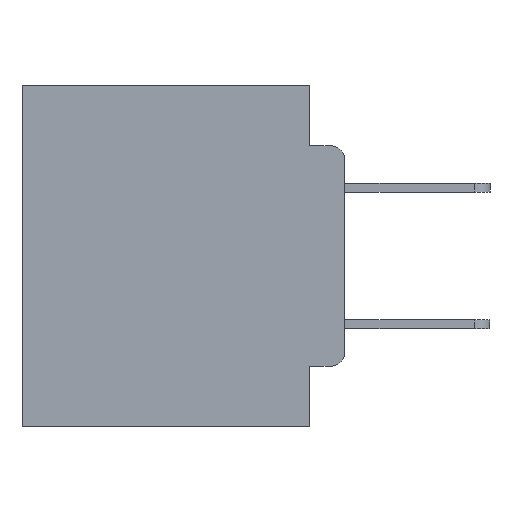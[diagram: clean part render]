
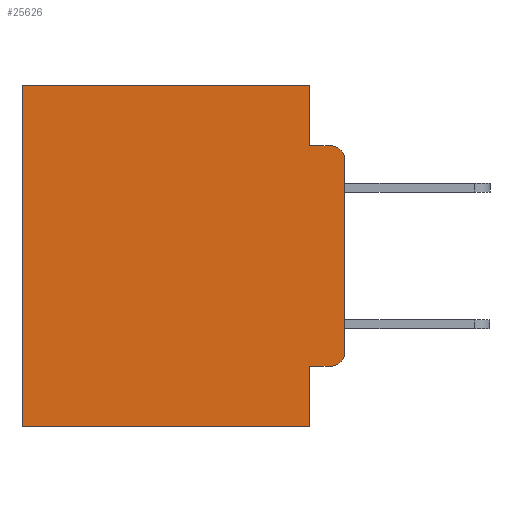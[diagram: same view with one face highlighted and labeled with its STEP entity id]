
A CAD part, left-side view. The second image highlights one B-rep face of the part: STEP entity #25626.
In plain terms, the highlighted planar face has unit normal (-1, 0, 0).
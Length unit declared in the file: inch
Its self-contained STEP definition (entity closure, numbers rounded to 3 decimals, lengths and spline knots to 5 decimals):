
#14 = VERTEX_POINT ( 'NONE', #15404 ) ;
#99 = CARTESIAN_POINT ( 'NONE',  ( 0.298, 0.473, 0. ) ) ;
#463 = EDGE_CURVE ( 'NONE', #4407, #11664, #24341, .T. ) ;
#512 = CARTESIAN_POINT ( 'NONE',  ( 0.298, 0.051, -0.0885 ) ) ;
#600 = ORIENTED_EDGE ( 'NONE', *, *, #10917, .T. ) ;
#1942 = CARTESIAN_POINT ( 'NONE',  ( 0.298, 0.051, -0.5 ) ) ;
#2270 = DIRECTION ( 'NONE',  ( 0., 0., -1. ) ) ;
#2298 = AXIS2_PLACEMENT_3D ( 'NONE', #17276, #5263, #19215 ) ;
#2495 = ORIENTED_EDGE ( 'NONE', *, *, #9375, .F. ) ;
#2598 = ORIENTED_EDGE ( 'NONE', *, *, #5978, .T. ) ;
#3048 = ORIENTED_EDGE ( 'NONE', *, *, #21684, .T. ) ;
#3461 = ORIENTED_EDGE ( 'NONE', *, *, #463, .F. ) ;
#3897 = VERTEX_POINT ( 'NONE', #512 ) ;
#4077 = LINE ( 'NONE', #16850, #19419 ) ;
#4146 = VERTEX_POINT ( 'NONE', #5907 ) ;
#4407 = VERTEX_POINT ( 'NONE', #6810 ) ;
#4542 = VECTOR ( 'NONE', #12290, 39.37008 ) ;
#5263 = DIRECTION ( 'NONE',  ( -1., 0., 0. ) ) ;
#5290 = CARTESIAN_POINT ( 'NONE',  ( 0.298, 0.02, -0.4115 ) ) ;
#5338 = ORIENTED_EDGE ( 'NONE', *, *, #9528, .T. ) ;
#5624 = ORIENTED_EDGE ( 'NONE', *, *, #22637, .F. ) ;
#5847 = ORIENTED_EDGE ( 'NONE', *, *, #11977, .F. ) ;
#5907 = CARTESIAN_POINT ( 'NONE',  ( 0.298, 0.051, -0.4115 ) ) ;
#5955 = ORIENTED_EDGE ( 'NONE', *, *, #23391, .T. ) ;
#5978 = EDGE_CURVE ( 'NONE', #4407, #24501, #9150, .T. ) ;
#6171 = VECTOR ( 'NONE', #20782, 39.37008 ) ;
#6336 = CARTESIAN_POINT ( 'NONE',  ( 0.298, 0.02, -0.1085 ) ) ;
#6393 = ORIENTED_EDGE ( 'NONE', *, *, #14927, .F. ) ;
#6546 = VECTOR ( 'NONE', #13984, 39.37008 ) ;
#6810 = CARTESIAN_POINT ( 'NONE',  ( 0.298, 0., -0.1085 ) ) ;
#6905 = CARTESIAN_POINT ( 'NONE',  ( 0.298, 0., -0.5 ) ) ;
#7185 = LINE ( 'NONE', #14065, #6546 ) ;
#7495 = CARTESIAN_POINT ( 'NONE',  ( 0.298, 0.02, -0.0885 ) ) ;
#7976 = CIRCLE ( 'NONE', #2298, 0.02 ) ;
#8357 = DIRECTION ( 'NONE',  ( 0., 0., -1. ) ) ;
#8379 = AXIS2_PLACEMENT_3D ( 'NONE', #17013, #9089, #22969 ) ;
#8479 = VECTOR ( 'NONE', #2270, 39.37008 ) ;
#8887 = CARTESIAN_POINT ( 'NONE',  ( 0.298, 0., 0. ) ) ;
#8903 = DIRECTION ( 'NONE',  ( 0., 0., -1. ) ) ;
#9089 = DIRECTION ( 'NONE',  ( 1., 0., 0. ) ) ;
#9150 = CIRCLE ( 'NONE', #14619, 0.02 ) ;
#9375 = EDGE_CURVE ( 'NONE', #19692, #14, #10938, .T. ) ;
#9528 = EDGE_CURVE ( 'NONE', #4146, #12264, #18308, .T. ) ;
#10236 = CARTESIAN_POINT ( 'NONE',  ( 0.298, 0.051, 0. ) ) ;
#10577 = DIRECTION ( 'NONE',  ( 0., 0., -1. ) ) ;
#10917 = EDGE_CURVE ( 'NONE', #12264, #11664, #7976, .T. ) ;
#10938 = LINE ( 'NONE', #6905, #6171 ) ;
#11664 = VERTEX_POINT ( 'NONE', #17562 ) ;
#11977 = EDGE_CURVE ( 'NONE', #13339, #3897, #13580, .T. ) ;
#12264 = VERTEX_POINT ( 'NONE', #5290 ) ;
#12290 = DIRECTION ( 'NONE',  ( 0., 0., -1. ) ) ;
#12565 = CARTESIAN_POINT ( 'NONE',  ( 0.298, 0.051, 0. ) ) ;
#13097 = VECTOR ( 'NONE', #15368, 39.37008 ) ;
#13339 = VERTEX_POINT ( 'NONE', #10236 ) ;
#13580 = LINE ( 'NONE', #12565, #23448 ) ;
#13984 = DIRECTION ( 'NONE',  ( 0., -1., 0. ) ) ;
#14065 = CARTESIAN_POINT ( 'NONE',  ( 0.298, 0.051, -0.0885 ) ) ;
#14271 = EDGE_LOOP ( 'NONE', ( #3461, #2598, #5624, #5847, #3048, #5955, #2495, #6393, #5338, #600 ) ) ;
#14619 = AXIS2_PLACEMENT_3D ( 'NONE', #6336, #20223, #8357 ) ;
#14927 = EDGE_CURVE ( 'NONE', #4146, #19692, #17165, .T. ) ;
#15368 = DIRECTION ( 'NONE',  ( 0., -1., 0. ) ) ;
#15404 = CARTESIAN_POINT ( 'NONE',  ( 0.298, 0.473, -0.5 ) ) ;
#16850 = CARTESIAN_POINT ( 'NONE',  ( 0.298, 0., 0. ) ) ;
#17013 = CARTESIAN_POINT ( 'NONE',  ( 0.298, 0., 0. ) ) ;
#17165 = LINE ( 'NONE', #20785, #17771 ) ;
#17276 = CARTESIAN_POINT ( 'NONE',  ( 0.298, 0.02, -0.3915 ) ) ;
#17562 = CARTESIAN_POINT ( 'NONE',  ( 0.298, 0., -0.3915 ) ) ;
#17771 = VECTOR ( 'NONE', #8903, 39.37008 ) ;
#17814 = CARTESIAN_POINT ( 'NONE',  ( 0.298, 0.473, 0. ) ) ;
#18029 = VERTEX_POINT ( 'NONE', #17814 ) ;
#18308 = LINE ( 'NONE', #23211, #13097 ) ;
#18784 = DIRECTION ( 'NONE',  ( 0., 1., 0. ) ) ;
#19215 = DIRECTION ( 'NONE',  ( 0., 0., -1. ) ) ;
#19419 = VECTOR ( 'NONE', #18784, 39.37008 ) ;
#19692 = VERTEX_POINT ( 'NONE', #1942 ) ;
#20223 = DIRECTION ( 'NONE',  ( -1., 0., 0. ) ) ;
#20782 = DIRECTION ( 'NONE',  ( 0., 1., 0. ) ) ;
#20785 = CARTESIAN_POINT ( 'NONE',  ( 0.298, 0.051, 0. ) ) ;
#21684 = EDGE_CURVE ( 'NONE', #13339, #18029, #4077, .T. ) ;
#22637 = EDGE_CURVE ( 'NONE', #3897, #24501, #7185, .T. ) ;
#22880 = PLANE ( 'NONE',  #8379 ) ;
#22969 = DIRECTION ( 'NONE',  ( 0., 0., -1. ) ) ;
#23211 = CARTESIAN_POINT ( 'NONE',  ( 0.298, 0.051, -0.4115 ) ) ;
#23391 = EDGE_CURVE ( 'NONE', #18029, #14, #25766, .T. ) ;
#23448 = VECTOR ( 'NONE', #10577, 39.37008 ) ;
#24341 = LINE ( 'NONE', #8887, #8479 ) ;
#24458 = FACE_OUTER_BOUND ( 'NONE', #14271, .T. ) ;
#24501 = VERTEX_POINT ( 'NONE', #7495 ) ;
#25626 = ADVANCED_FACE ( 'NONE', ( #24458 ), #22880, .F. ) ;
#25766 = LINE ( 'NONE', #99, #4542 ) ;
